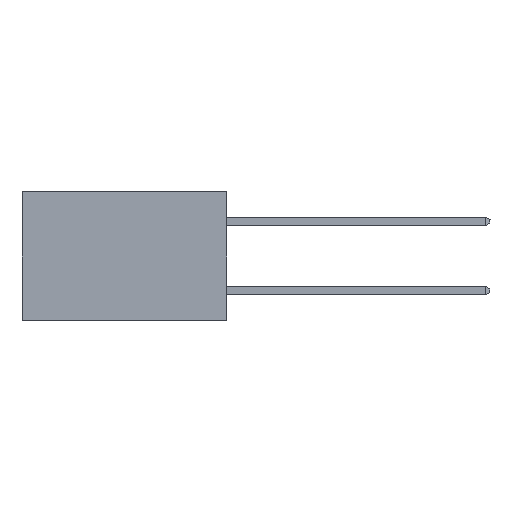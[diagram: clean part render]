
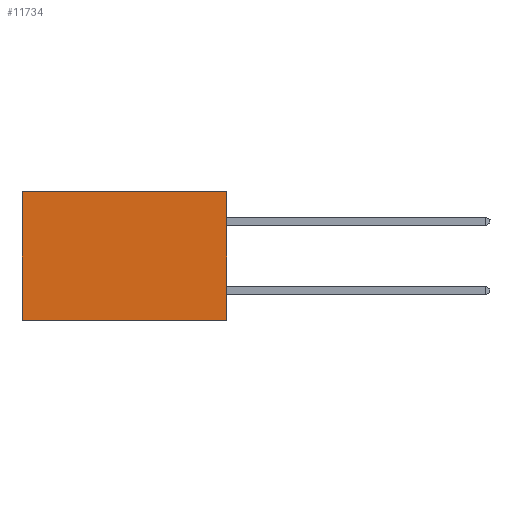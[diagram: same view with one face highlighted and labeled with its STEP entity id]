
A CAD part, left-side view. The second image highlights one B-rep face of the part: STEP entity #11734.
In plain terms, the highlighted planar face has unit normal (-1, 0, 0).
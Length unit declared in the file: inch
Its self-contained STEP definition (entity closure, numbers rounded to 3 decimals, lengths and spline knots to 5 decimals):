
#468 = ORIENTED_EDGE ( 'NONE', *, *, #2412, .T. ) ;
#1559 = EDGE_CURVE ( 'NONE', #13207, #10894, #5525, .T. ) ;
#1712 = EDGE_LOOP ( 'NONE', ( #468, #6825, #20098, #21548 ) ) ;
#2412 = EDGE_CURVE ( 'NONE', #10169, #10894, #14041, .T. ) ;
#3185 = EDGE_CURVE ( 'NONE', #27399, #10169, #17632, .T. ) ;
#3778 = CARTESIAN_POINT ( 'NONE',  ( 0.277, 0., -0.37 ) ) ;
#5525 = LINE ( 'NONE', #3778, #29588 ) ;
#6713 = DIRECTION ( 'NONE',  ( 0., 0., -1. ) ) ;
#6761 = LINE ( 'NONE', #21539, #19287 ) ;
#6825 = ORIENTED_EDGE ( 'NONE', *, *, #1559, .F. ) ;
#7731 = VECTOR ( 'NONE', #6713, 39.37008 ) ;
#7773 = CARTESIAN_POINT ( 'NONE',  ( 0.277, 0.59, -0.37 ) ) ;
#8434 = DIRECTION ( 'NONE',  ( 1., 0., 0. ) ) ;
#9843 = DIRECTION ( 'NONE',  ( 0., 0., -1. ) ) ;
#9932 = CARTESIAN_POINT ( 'NONE',  ( 0.277, 0., 0. ) ) ;
#10031 = DIRECTION ( 'NONE',  ( 0., 1., 0. ) ) ;
#10169 = VERTEX_POINT ( 'NONE', #23643 ) ;
#10733 = CARTESIAN_POINT ( 'NONE',  ( 0.277, 0., -0.37 ) ) ;
#10894 = VERTEX_POINT ( 'NONE', #15207 ) ;
#11413 = VECTOR ( 'NONE', #10031, 39.37008 ) ;
#11734 = ADVANCED_FACE ( 'NONE', ( #24742 ), #20165, .F. ) ;
#13207 = VERTEX_POINT ( 'NONE', #13376 ) ;
#13376 = CARTESIAN_POINT ( 'NONE',  ( 0.277, 0., -0.37 ) ) ;
#14041 = LINE ( 'NONE', #7773, #7731 ) ;
#15207 = CARTESIAN_POINT ( 'NONE',  ( 0.277, 0.59, -0.37 ) ) ;
#15272 = AXIS2_PLACEMENT_3D ( 'NONE', #10733, #8434, #24844 ) ;
#17632 = LINE ( 'NONE', #9932, #11413 ) ;
#19287 = VECTOR ( 'NONE', #9843, 39.37008 ) ;
#20098 = ORIENTED_EDGE ( 'NONE', *, *, #24165, .F. ) ;
#20165 = PLANE ( 'NONE',  #15272 ) ;
#21539 = CARTESIAN_POINT ( 'NONE',  ( 0.277, 0., -0.37 ) ) ;
#21548 = ORIENTED_EDGE ( 'NONE', *, *, #3185, .T. ) ;
#22673 = DIRECTION ( 'NONE',  ( 0., 1., 0. ) ) ;
#23643 = CARTESIAN_POINT ( 'NONE',  ( 0.277, 0.59, 0. ) ) ;
#24165 = EDGE_CURVE ( 'NONE', #27399, #13207, #6761, .T. ) ;
#24742 = FACE_OUTER_BOUND ( 'NONE', #1712, .T. ) ;
#24844 = DIRECTION ( 'NONE',  ( 0., 0., -1. ) ) ;
#27399 = VERTEX_POINT ( 'NONE', #29511 ) ;
#29511 = CARTESIAN_POINT ( 'NONE',  ( 0.277, 0., 0. ) ) ;
#29588 = VECTOR ( 'NONE', #22673, 39.37008 ) ;
